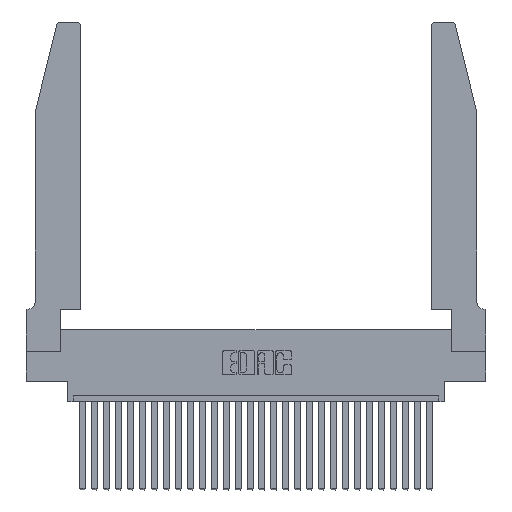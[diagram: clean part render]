
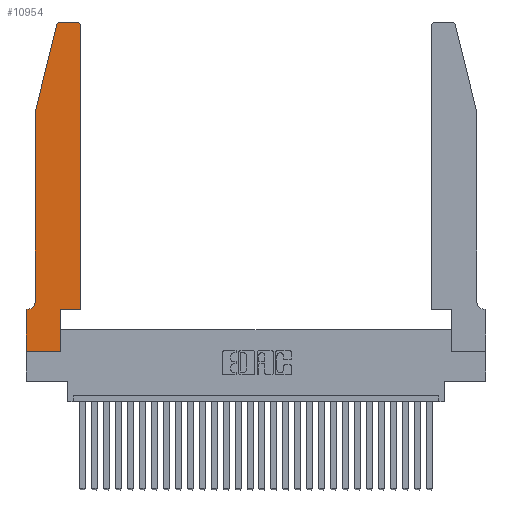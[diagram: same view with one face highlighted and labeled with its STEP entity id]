
A CAD part, top view. The second image highlights one B-rep face of the part: STEP entity #10954.
In plain terms, the highlighted planar face has unit normal (0, 0, 1).
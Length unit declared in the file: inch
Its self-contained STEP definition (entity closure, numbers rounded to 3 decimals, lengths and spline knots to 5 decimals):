
#342 = LINE ( 'NONE', #18341, #17512 ) ;
#1099 = EDGE_CURVE ( 'NONE', #12147, #7852, #6385, .T. ) ;
#1760 = LINE ( 'NONE', #13461, #24805 ) ;
#1967 = ORIENTED_EDGE ( 'NONE', *, *, #25930, .T. ) ;
#2536 = ORIENTED_EDGE ( 'NONE', *, *, #19378, .T. ) ;
#2565 = CIRCLE ( 'NONE', #27728, 0.03 ) ;
#2699 = DIRECTION ( 'NONE',  ( 0., -1., 0. ) ) ;
#2951 = EDGE_CURVE ( 'NONE', #15497, #6914, #21953, .T. ) ;
#3415 = FACE_OUTER_BOUND ( 'NONE', #15240, .T. ) ;
#3536 = VERTEX_POINT ( 'NONE', #17317 ) ;
#3916 = EDGE_CURVE ( 'NONE', #6914, #5672, #26738, .T. ) ;
#4001 = CARTESIAN_POINT ( 'NONE',  ( 0.0755, 2., 0.37 ) ) ;
#5261 = ORIENTED_EDGE ( 'NONE', *, *, #1099, .T. ) ;
#5672 = VERTEX_POINT ( 'NONE', #25625 ) ;
#5720 = CARTESIAN_POINT ( 'NONE',  ( 0.2865, 0.35, 0.37 ) ) ;
#6079 = CARTESIAN_POINT ( 'NONE',  ( 0.0755, 2., 0.37 ) ) ;
#6106 = CARTESIAN_POINT ( 'NONE',  ( 0.4205, 2.72, 0.37 ) ) ;
#6129 = ORIENTED_EDGE ( 'NONE', *, *, #12686, .T. ) ;
#6223 = CARTESIAN_POINT ( 'NONE',  ( 0.0755, 2., 0.37 ) ) ;
#6385 = LINE ( 'NONE', #15431, #27969 ) ;
#6474 = CARTESIAN_POINT ( 'NONE',  ( 0.4505, 0.35, 0.37 ) ) ;
#6481 = CARTESIAN_POINT ( 'NONE',  ( 0., 0., 0.37 ) ) ;
#6556 = CARTESIAN_POINT ( 'NONE',  ( 0.0755, 0.42, 0.37 ) ) ;
#6691 = LINE ( 'NONE', #22824, #25169 ) ;
#6914 = VERTEX_POINT ( 'NONE', #6556 ) ;
#7252 = ORIENTED_EDGE ( 'NONE', *, *, #22909, .T. ) ;
#7333 = VERTEX_POINT ( 'NONE', #27956 ) ;
#7395 = VECTOR ( 'NONE', #28642, 39.37008 ) ;
#7852 = VERTEX_POINT ( 'NONE', #24831 ) ;
#8049 = EDGE_CURVE ( 'NONE', #14123, #3536, #18160, .T. ) ;
#9091 = DIRECTION ( 'NONE',  ( 1., 0., 0. ) ) ;
#9488 = DIRECTION ( 'NONE',  ( 1., 0., 0. ) ) ;
#9567 = ORIENTED_EDGE ( 'NONE', *, *, #8049, .T. ) ;
#10954 = ADVANCED_FACE ( 'NONE', ( #3415 ), #20775, .T. ) ;
#11144 = DIRECTION ( 'NONE',  ( 0., 1., 0. ) ) ;
#11913 = CARTESIAN_POINT ( 'NONE',  ( 0., 0.35, 0.37 ) ) ;
#12142 = ORIENTED_EDGE ( 'NONE', *, *, #20184, .T. ) ;
#12147 = VERTEX_POINT ( 'NONE', #14128 ) ;
#12193 = DIRECTION ( 'NONE',  ( 1., 0., 0. ) ) ;
#12686 = EDGE_CURVE ( 'NONE', #23485, #7333, #24936, .T. ) ;
#12802 = DIRECTION ( 'NONE',  ( -0.239, -0.971, 0. ) ) ;
#13117 = VECTOR ( 'NONE', #11144, 39.37008 ) ;
#13461 = CARTESIAN_POINT ( 'NONE',  ( 0.2865, 0.35, 0.37 ) ) ;
#14123 = VERTEX_POINT ( 'NONE', #17438 ) ;
#14128 = CARTESIAN_POINT ( 'NONE',  ( 0.4205, 2.75, 0.37 ) ) ;
#14676 = VERTEX_POINT ( 'NONE', #5720 ) ;
#15020 = AXIS2_PLACEMENT_3D ( 'NONE', #18626, #27574, #18932 ) ;
#15240 = EDGE_LOOP ( 'NONE', ( #5261, #2536, #25981, #24163, #25573, #27382, #9567, #7252, #1967, #19406, #6129, #12142 ) ) ;
#15431 = CARTESIAN_POINT ( 'NONE',  ( 0.2605, 2.75, 0.37 ) ) ;
#15497 = VERTEX_POINT ( 'NONE', #6223 ) ;
#15780 = CARTESIAN_POINT ( 'NONE',  ( 0.25487, 2.72718, 0.37 ) ) ;
#15951 = DIRECTION ( 'NONE',  ( 0., 0., 1. ) ) ;
#15992 = DIRECTION ( 'NONE',  ( -1., 0., 0. ) ) ;
#16019 = AXIS2_PLACEMENT_3D ( 'NONE', #11913, #25831, #16713 ) ;
#16052 = CARTESIAN_POINT ( 'NONE',  ( 0.284, 2.72, 0.37 ) ) ;
#16713 = DIRECTION ( 'NONE',  ( 1., 0., 0. ) ) ;
#17317 = CARTESIAN_POINT ( 'NONE',  ( 0., 0., 0.37 ) ) ;
#17438 = CARTESIAN_POINT ( 'NONE',  ( 0., 0.35, 0.37 ) ) ;
#17512 = VECTOR ( 'NONE', #22663, 39.37008 ) ;
#17535 = CIRCLE ( 'NONE', #22161, 0.03 ) ;
#18077 = VECTOR ( 'NONE', #2699, 39.37008 ) ;
#18160 = LINE ( 'NONE', #26312, #7395 ) ;
#18242 = DIRECTION ( 'NONE',  ( 1., 0., 0. ) ) ;
#18341 = CARTESIAN_POINT ( 'NONE',  ( 0.0755, 0.35, 0.37 ) ) ;
#18626 = CARTESIAN_POINT ( 'NONE',  ( 0.0055, 0.42, 0.37 ) ) ;
#18932 = DIRECTION ( 'NONE',  ( -1., 0., 0. ) ) ;
#19378 = EDGE_CURVE ( 'NONE', #7852, #27658, #2565, .T. ) ;
#19406 = ORIENTED_EDGE ( 'NONE', *, *, #20776, .T. ) ;
#19560 = CARTESIAN_POINT ( 'NONE',  ( 0.2865, 0., 0.37 ) ) ;
#20099 = DIRECTION ( 'NONE',  ( 0., 0., 1. ) ) ;
#20184 = EDGE_CURVE ( 'NONE', #7333, #12147, #17535, .T. ) ;
#20529 = EDGE_CURVE ( 'NONE', #5672, #14123, #342, .T. ) ;
#20775 = PLANE ( 'NONE',  #16019 ) ;
#20776 = EDGE_CURVE ( 'NONE', #14676, #23485, #6691, .T. ) ;
#21907 = VECTOR ( 'NONE', #12193, 39.37008 ) ;
#21953 = LINE ( 'NONE', #4001, #18077 ) ;
#22161 = AXIS2_PLACEMENT_3D ( 'NONE', #6106, #20099, #9091 ) ;
#22663 = DIRECTION ( 'NONE',  ( -1., 0., 0. ) ) ;
#22744 = VERTEX_POINT ( 'NONE', #19560 ) ;
#22824 = CARTESIAN_POINT ( 'NONE',  ( 0.4505, 0.35, 0.37 ) ) ;
#22909 = EDGE_CURVE ( 'NONE', #3536, #22744, #27816, .T. ) ;
#23485 = VERTEX_POINT ( 'NONE', #26701 ) ;
#23705 = VECTOR ( 'NONE', #12802, 39.37008 ) ;
#24163 = ORIENTED_EDGE ( 'NONE', *, *, #2951, .T. ) ;
#24805 = VECTOR ( 'NONE', #26853, 39.37008 ) ;
#24831 = CARTESIAN_POINT ( 'NONE',  ( 0.284, 2.75, 0.37 ) ) ;
#24936 = LINE ( 'NONE', #6474, #13117 ) ;
#25169 = VECTOR ( 'NONE', #9488, 39.37008 ) ;
#25573 = ORIENTED_EDGE ( 'NONE', *, *, #3916, .T. ) ;
#25625 = CARTESIAN_POINT ( 'NONE',  ( 0.0055, 0.35, 0.37 ) ) ;
#25831 = DIRECTION ( 'NONE',  ( 0., 0., 1. ) ) ;
#25930 = EDGE_CURVE ( 'NONE', #22744, #14676, #1760, .T. ) ;
#25981 = ORIENTED_EDGE ( 'NONE', *, *, #27414, .T. ) ;
#26312 = CARTESIAN_POINT ( 'NONE',  ( 0., 0., 0.37 ) ) ;
#26701 = CARTESIAN_POINT ( 'NONE',  ( 0.4505, 0.35, 0.37 ) ) ;
#26738 = CIRCLE ( 'NONE', #15020, 0.07 ) ;
#26853 = DIRECTION ( 'NONE',  ( 0., 1., 0. ) ) ;
#27160 = LINE ( 'NONE', #6079, #23705 ) ;
#27382 = ORIENTED_EDGE ( 'NONE', *, *, #20529, .T. ) ;
#27414 = EDGE_CURVE ( 'NONE', #27658, #15497, #27160, .T. ) ;
#27574 = DIRECTION ( 'NONE',  ( 0., 0., -1. ) ) ;
#27658 = VERTEX_POINT ( 'NONE', #15780 ) ;
#27728 = AXIS2_PLACEMENT_3D ( 'NONE', #16052, #15951, #18242 ) ;
#27816 = LINE ( 'NONE', #6481, #21907 ) ;
#27956 = CARTESIAN_POINT ( 'NONE',  ( 0.4505, 2.72, 0.37 ) ) ;
#27969 = VECTOR ( 'NONE', #15992, 39.37008 ) ;
#28642 = DIRECTION ( 'NONE',  ( 0., -1., 0. ) ) ;
